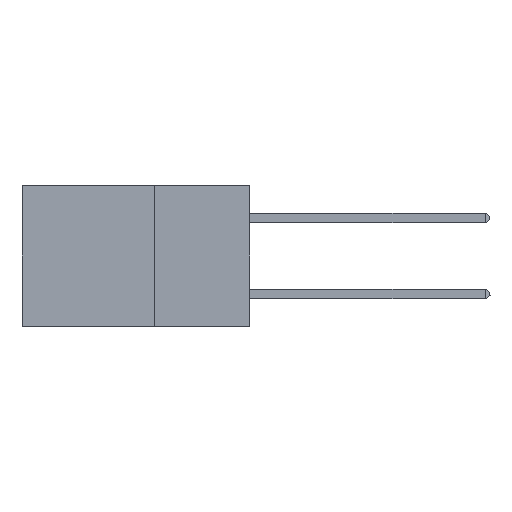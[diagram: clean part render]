
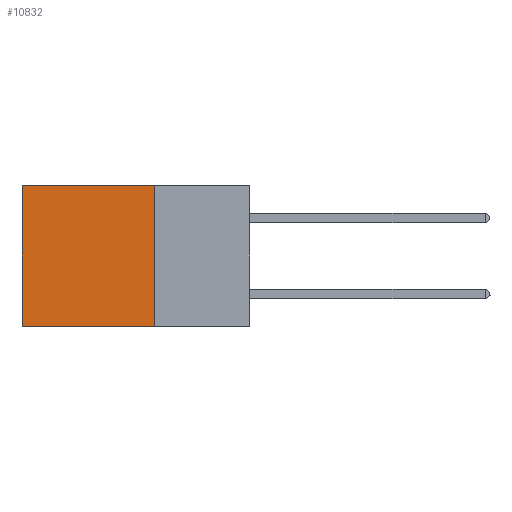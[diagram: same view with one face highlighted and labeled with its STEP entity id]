
A CAD part, left-side view. The second image highlights one B-rep face of the part: STEP entity #10832.
In plain terms, the highlighted planar face has unit normal (-1, 0, 0).
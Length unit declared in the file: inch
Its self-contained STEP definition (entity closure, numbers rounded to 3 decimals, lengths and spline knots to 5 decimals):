
#237 = PLANE ( 'NONE',  #18326 ) ;
#1279 = DIRECTION ( 'NONE',  ( 0., 0., -1. ) ) ;
#1687 = DIRECTION ( 'NONE',  ( 0., 0., -1. ) ) ;
#2036 = EDGE_CURVE ( 'NONE', #16391, #18104, #16567, .T. ) ;
#2416 = EDGE_CURVE ( 'NONE', #10834, #7099, #3696, .T. ) ;
#3696 = LINE ( 'NONE', #13755, #17894 ) ;
#4073 = VECTOR ( 'NONE', #17767, 39.37008 ) ;
#4206 = CARTESIAN_POINT ( 'NONE',  ( 0.2875, 0.25, 0. ) ) ;
#4460 = ORIENTED_EDGE ( 'NONE', *, *, #2416, .T. ) ;
#4635 = CARTESIAN_POINT ( 'NONE',  ( 0.2875, 0.25, 0. ) ) ;
#4696 = EDGE_CURVE ( 'NONE', #16391, #10834, #16468, .T. ) ;
#5635 = ORIENTED_EDGE ( 'NONE', *, *, #2036, .F. ) ;
#5956 = CARTESIAN_POINT ( 'NONE',  ( 0.2875, 0.25, 0. ) ) ;
#6290 = ORIENTED_EDGE ( 'NONE', *, *, #10844, .F. ) ;
#7099 = VERTEX_POINT ( 'NONE', #16851 ) ;
#7658 = LINE ( 'NONE', #17679, #11289 ) ;
#8268 = ORIENTED_EDGE ( 'NONE', *, *, #4696, .T. ) ;
#8523 = CARTESIAN_POINT ( 'NONE',  ( 0.2875, 0.25, -0.37 ) ) ;
#10364 = CARTESIAN_POINT ( 'NONE',  ( 0.2875, 0.6, 0. ) ) ;
#10426 = DIRECTION ( 'NONE',  ( 1., 0., 0. ) ) ;
#10832 = ADVANCED_FACE ( 'NONE', ( #18298 ), #237, .F. ) ;
#10834 = VERTEX_POINT ( 'NONE', #10364 ) ;
#10844 = EDGE_CURVE ( 'NONE', #18104, #7099, #7658, .T. ) ;
#11289 = VECTOR ( 'NONE', #14626, 39.37008 ) ;
#12287 = VECTOR ( 'NONE', #1279, 39.37008 ) ;
#12494 = DIRECTION ( 'NONE',  ( 0., 0., -1. ) ) ;
#13755 = CARTESIAN_POINT ( 'NONE',  ( 0.2875, 0.6, 0. ) ) ;
#14040 = EDGE_LOOP ( 'NONE', ( #4460, #6290, #5635, #8268 ) ) ;
#14626 = DIRECTION ( 'NONE',  ( 0., 1., 0. ) ) ;
#16391 = VERTEX_POINT ( 'NONE', #5956 ) ;
#16440 = CARTESIAN_POINT ( 'NONE',  ( 0.2875, 0.25, 0. ) ) ;
#16468 = LINE ( 'NONE', #16440, #4073 ) ;
#16567 = LINE ( 'NONE', #4206, #12287 ) ;
#16851 = CARTESIAN_POINT ( 'NONE',  ( 0.2875, 0.6, -0.37 ) ) ;
#17679 = CARTESIAN_POINT ( 'NONE',  ( 0.2875, 0.25, -0.37 ) ) ;
#17767 = DIRECTION ( 'NONE',  ( 0., 1., 0. ) ) ;
#17894 = VECTOR ( 'NONE', #12494, 39.37008 ) ;
#18104 = VERTEX_POINT ( 'NONE', #8523 ) ;
#18298 = FACE_OUTER_BOUND ( 'NONE', #14040, .T. ) ;
#18326 = AXIS2_PLACEMENT_3D ( 'NONE', #4635, #10426, #1687 ) ;
